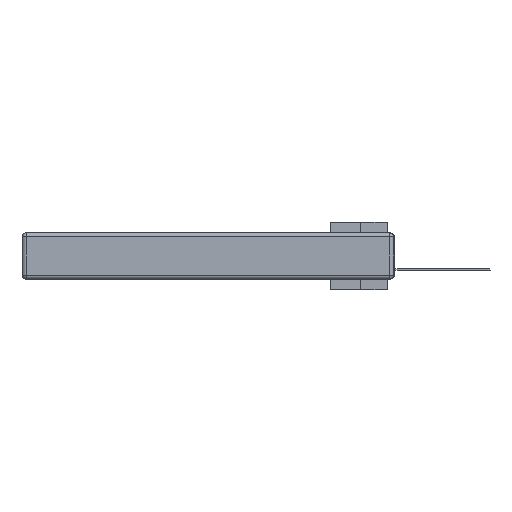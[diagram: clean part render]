
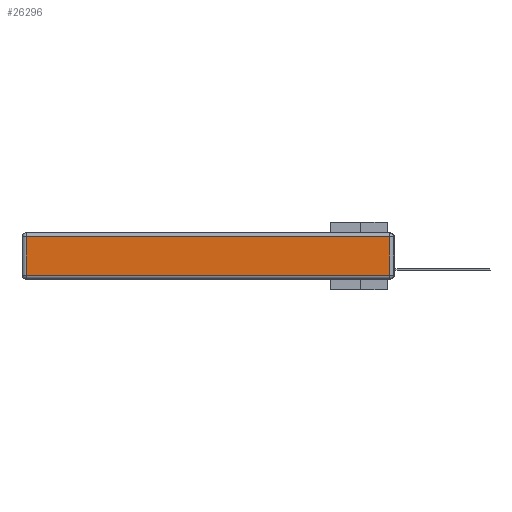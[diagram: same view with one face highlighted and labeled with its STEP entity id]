
A CAD part, left-side view. The second image highlights one B-rep face of the part: STEP entity #26296.
In plain terms, the highlighted planar face has unit normal (-1, 0, 0).
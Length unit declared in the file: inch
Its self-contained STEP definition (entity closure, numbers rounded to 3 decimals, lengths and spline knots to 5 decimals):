
#469 = EDGE_CURVE ( 'NONE', #22199, #24786, #624, .T. ) ;
#624 = LINE ( 'NONE', #29980, #21362 ) ;
#1171 = DIRECTION ( 'NONE',  ( 0., -1., 0. ) ) ;
#1279 = VECTOR ( 'NONE', #5258, 39.37008 ) ;
#1902 = EDGE_CURVE ( 'NONE', #14291, #22199, #7169, .T. ) ;
#2613 = CARTESIAN_POINT ( 'NONE',  ( 0., 2.75, -0.03 ) ) ;
#2877 = ORIENTED_EDGE ( 'NONE', *, *, #20866, .T. ) ;
#3763 = LINE ( 'NONE', #2613, #1279 ) ;
#3855 = VERTEX_POINT ( 'NONE', #10921 ) ;
#5258 = DIRECTION ( 'NONE',  ( 0., 1., 0. ) ) ;
#5878 = DIRECTION ( 'NONE',  ( 0., 0., 1. ) ) ;
#6481 = EDGE_LOOP ( 'NONE', ( #13039, #2877, #24494, #19086 ) ) ;
#7169 = LINE ( 'NONE', #10408, #26277 ) ;
#8365 = CARTESIAN_POINT ( 'NONE',  ( 0., 0.03, -0.343 ) ) ;
#10408 = CARTESIAN_POINT ( 'NONE',  ( 0., 2.72, -0.343 ) ) ;
#10921 = CARTESIAN_POINT ( 'NONE',  ( 0., 0.03, -0.03 ) ) ;
#10957 = PLANE ( 'NONE',  #14795 ) ;
#11203 = EDGE_CURVE ( 'NONE', #3855, #14291, #3763, .T. ) ;
#13039 = ORIENTED_EDGE ( 'NONE', *, *, #469, .T. ) ;
#14291 = VERTEX_POINT ( 'NONE', #17730 ) ;
#14381 = CARTESIAN_POINT ( 'NONE',  ( 0., 2.72, -0.313 ) ) ;
#14795 = AXIS2_PLACEMENT_3D ( 'NONE', #27084, #21537, #5878 ) ;
#16356 = DIRECTION ( 'NONE',  ( 0., 0., 1. ) ) ;
#17730 = CARTESIAN_POINT ( 'NONE',  ( 0., 2.72, -0.03 ) ) ;
#19086 = ORIENTED_EDGE ( 'NONE', *, *, #1902, .T. ) ;
#20560 = VECTOR ( 'NONE', #16356, 39.37008 ) ;
#20866 = EDGE_CURVE ( 'NONE', #24786, #3855, #21373, .T. ) ;
#21362 = VECTOR ( 'NONE', #1171, 39.37008 ) ;
#21373 = LINE ( 'NONE', #8365, #20560 ) ;
#21537 = DIRECTION ( 'NONE',  ( -1., 0., 0. ) ) ;
#22199 = VERTEX_POINT ( 'NONE', #14381 ) ;
#23931 = FACE_OUTER_BOUND ( 'NONE', #6481, .T. ) ;
#24494 = ORIENTED_EDGE ( 'NONE', *, *, #11203, .T. ) ;
#24786 = VERTEX_POINT ( 'NONE', #25796 ) ;
#25796 = CARTESIAN_POINT ( 'NONE',  ( 0., 0.03, -0.313 ) ) ;
#25994 = DIRECTION ( 'NONE',  ( 0., 0., -1. ) ) ;
#26277 = VECTOR ( 'NONE', #25994, 39.37008 ) ;
#26296 = ADVANCED_FACE ( 'NONE', ( #23931 ), #10957, .T. ) ;
#27084 = CARTESIAN_POINT ( 'NONE',  ( 0., 0., -0.343 ) ) ;
#29980 = CARTESIAN_POINT ( 'NONE',  ( 0., 0., -0.313 ) ) ;
